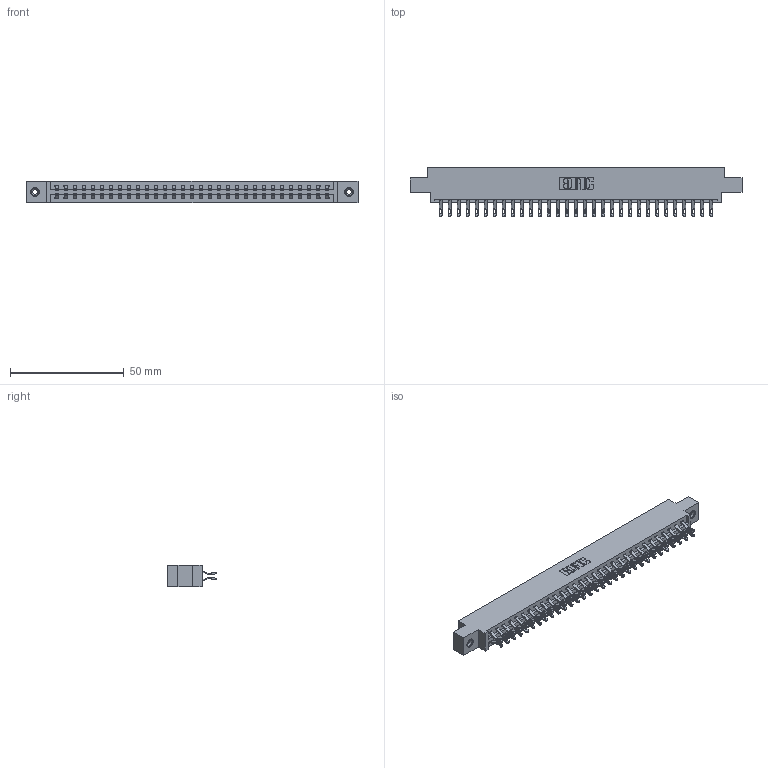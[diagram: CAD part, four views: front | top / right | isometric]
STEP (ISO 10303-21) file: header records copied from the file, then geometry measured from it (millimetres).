
FILE_DESCRIPTION (( 'STEP AP203' ), '1' );
FILE_NAME ('337-062-555-808.STEP', '2018-08-11T04:38:13', ( '' ), ( '' ), 'SwSTEP 2.0', 'SolidWorks 2016', '' );
FILE_SCHEMA (( 'CONFIG_CONTROL_DESIGN' ));
Length unit declared in the file: inch
Products named in the file (4): 345-292-001_555 Tail; 345-250-001_345-250-003-102; 337-062-555-808; 337 Part_0.170 Offset - 0.156 Dia-TI
Assembly tree (65 placements, depth 2):
  337-062-555-808
    337 Part_0.170 Offset - 0.156 Dia-TI
    345-292-001_555 Tail  x62
    345-250-001_345-250-003-102  x2
Bounding box: 145.85 x 21.47 x 9.4 mm (x, y, z)
Volume: 15279.9 mm3; surface area: 17976.6 mm2
Topology: 65 solids, 65 shells, 3898 faces, 12177 edges, 8110 vertices
Faces by surface type: plane 2338, cylinder 1544, cone 12, torus 4
Entity records: 27102 total; most frequent: CARTESIAN_POINT 4591, ORIENTED_EDGE 4490, DIRECTION 3927, EDGE_CURVE 2245, LINE 2077, VECTOR 2077, VERTEX_POINT 1492, AXIS2_PLACEMENT_3D 925
